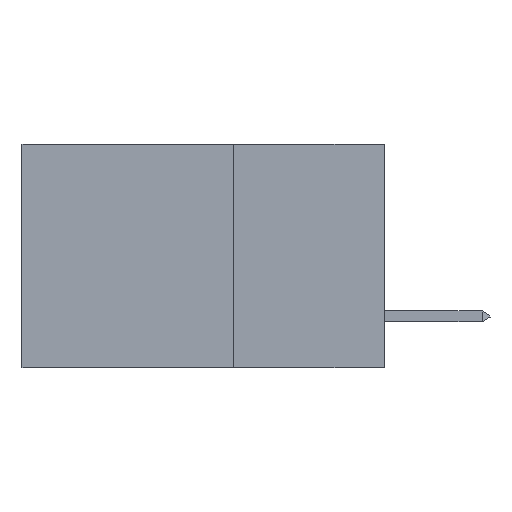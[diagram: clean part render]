
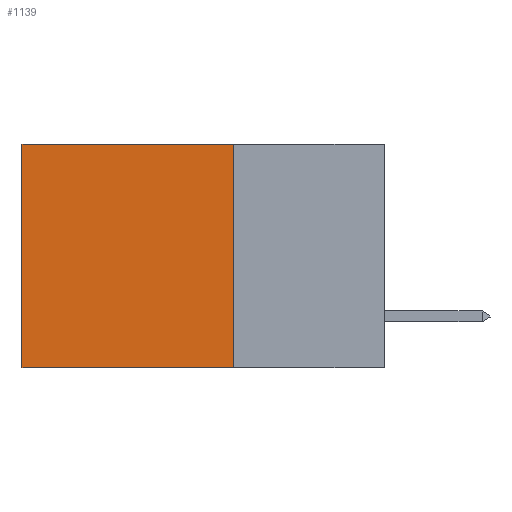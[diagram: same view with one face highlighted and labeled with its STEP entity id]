
A CAD part, left-side view. The second image highlights one B-rep face of the part: STEP entity #1139.
In plain terms, the highlighted planar face has unit normal (-1, 0, 0).
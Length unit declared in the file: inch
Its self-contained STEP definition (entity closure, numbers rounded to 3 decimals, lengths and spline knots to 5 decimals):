
#801 = VECTOR ( 'NONE', #16509, 39.37008 ) ;
#933 = CARTESIAN_POINT ( 'NONE',  ( 0.2875, 0.6, 0. ) ) ;
#1139 = ADVANCED_FACE ( 'NONE', ( #16575 ), #1511, .F. ) ;
#1313 = ORIENTED_EDGE ( 'NONE', *, *, #2537, .T. ) ;
#1511 = PLANE ( 'NONE',  #24287 ) ;
#1719 = CARTESIAN_POINT ( 'NONE',  ( 0.2875, 0.25, -0.37 ) ) ;
#2537 = EDGE_CURVE ( 'NONE', #13539, #5261, #7355, .T. ) ;
#3234 = CARTESIAN_POINT ( 'NONE',  ( 0.2875, 0.25, 0. ) ) ;
#4230 = CARTESIAN_POINT ( 'NONE',  ( 0.2875, 0.6, 0. ) ) ;
#4733 = DIRECTION ( 'NONE',  ( 0., 0., -1. ) ) ;
#5261 = VERTEX_POINT ( 'NONE', #13379 ) ;
#5666 = DIRECTION ( 'NONE',  ( 0., 1., 0. ) ) ;
#6671 = CARTESIAN_POINT ( 'NONE',  ( 0.2875, 0.25, -0.37 ) ) ;
#6900 = VERTEX_POINT ( 'NONE', #18121 ) ;
#7041 = DIRECTION ( 'NONE',  ( 1., 0., 0. ) ) ;
#7355 = LINE ( 'NONE', #4230, #12246 ) ;
#10314 = VERTEX_POINT ( 'NONE', #1719 ) ;
#11457 = LINE ( 'NONE', #21603, #16643 ) ;
#11744 = ORIENTED_EDGE ( 'NONE', *, *, #16932, .F. ) ;
#12067 = LINE ( 'NONE', #23594, #18558 ) ;
#12246 = VECTOR ( 'NONE', #21877, 39.37008 ) ;
#13379 = CARTESIAN_POINT ( 'NONE',  ( 0.2875, 0.6, -0.37 ) ) ;
#13539 = VERTEX_POINT ( 'NONE', #933 ) ;
#14237 = EDGE_LOOP ( 'NONE', ( #1313, #11744, #17348, #22399 ) ) ;
#16476 = LINE ( 'NONE', #6671, #801 ) ;
#16509 = DIRECTION ( 'NONE',  ( 0., 1., 0. ) ) ;
#16575 = FACE_OUTER_BOUND ( 'NONE', #14237, .T. ) ;
#16643 = VECTOR ( 'NONE', #4733, 39.37008 ) ;
#16932 = EDGE_CURVE ( 'NONE', #10314, #5261, #16476, .T. ) ;
#17348 = ORIENTED_EDGE ( 'NONE', *, *, #25045, .F. ) ;
#18121 = CARTESIAN_POINT ( 'NONE',  ( 0.2875, 0.25, 0. ) ) ;
#18558 = VECTOR ( 'NONE', #5666, 39.37008 ) ;
#20402 = EDGE_CURVE ( 'NONE', #6900, #13539, #12067, .T. ) ;
#20841 = DIRECTION ( 'NONE',  ( 0., 0., -1. ) ) ;
#21603 = CARTESIAN_POINT ( 'NONE',  ( 0.2875, 0.25, 0. ) ) ;
#21877 = DIRECTION ( 'NONE',  ( 0., 0., -1. ) ) ;
#22399 = ORIENTED_EDGE ( 'NONE', *, *, #20402, .T. ) ;
#23594 = CARTESIAN_POINT ( 'NONE',  ( 0.2875, 0.25, 0. ) ) ;
#24287 = AXIS2_PLACEMENT_3D ( 'NONE', #3234, #7041, #20841 ) ;
#25045 = EDGE_CURVE ( 'NONE', #6900, #10314, #11457, .T. ) ;
